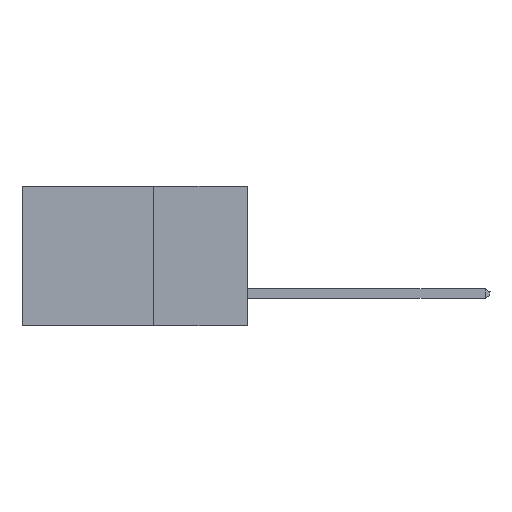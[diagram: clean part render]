
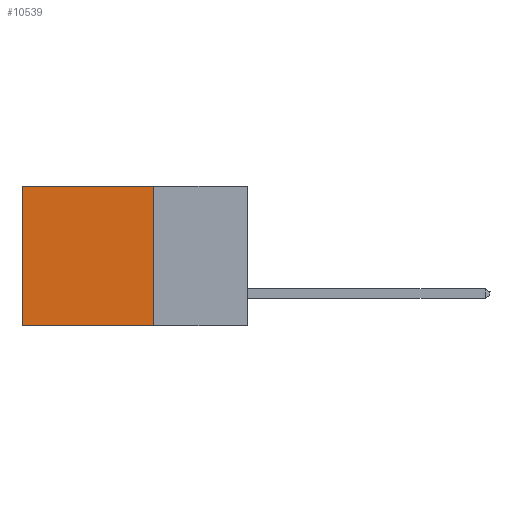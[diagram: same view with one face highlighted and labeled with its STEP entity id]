
A CAD part, left-side view. The second image highlights one B-rep face of the part: STEP entity #10539.
In plain terms, the highlighted planar face has unit normal (-1, 0, 0).
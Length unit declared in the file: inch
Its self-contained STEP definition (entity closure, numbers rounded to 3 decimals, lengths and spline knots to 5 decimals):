
#1441 = CARTESIAN_POINT ( 'NONE',  ( 0.2615, 0.25, -0.37 ) ) ;
#1574 = EDGE_CURVE ( 'NONE', #5538, #5189, #11603, .T. ) ;
#1950 = EDGE_CURVE ( 'NONE', #5538, #12675, #4213, .T. ) ;
#2228 = EDGE_LOOP ( 'NONE', ( #14907, #11228, #4739, #11250 ) ) ;
#2386 = FACE_OUTER_BOUND ( 'NONE', #2228, .T. ) ;
#3394 = CARTESIAN_POINT ( 'NONE',  ( 0.2615, 0.25, 0. ) ) ;
#4213 = LINE ( 'NONE', #5120, #4455 ) ;
#4455 = VECTOR ( 'NONE', #9991, 39.37008 ) ;
#4698 = DIRECTION ( 'NONE',  ( 0., 0., -1. ) ) ;
#4739 = ORIENTED_EDGE ( 'NONE', *, *, #1574, .F. ) ;
#5120 = CARTESIAN_POINT ( 'NONE',  ( 0.2615, 0.25, 0. ) ) ;
#5189 = VERTEX_POINT ( 'NONE', #6951 ) ;
#5538 = VERTEX_POINT ( 'NONE', #3394 ) ;
#6951 = CARTESIAN_POINT ( 'NONE',  ( 0.2615, 0.25, -0.37 ) ) ;
#7607 = DIRECTION ( 'NONE',  ( 0., 1., 0. ) ) ;
#7845 = VERTEX_POINT ( 'NONE', #7915 ) ;
#7915 = CARTESIAN_POINT ( 'NONE',  ( 0.2615, 0.6, -0.37 ) ) ;
#8578 = LINE ( 'NONE', #14483, #9137 ) ;
#9137 = VECTOR ( 'NONE', #10719, 39.37008 ) ;
#9604 = AXIS2_PLACEMENT_3D ( 'NONE', #10703, #13439, #4698 ) ;
#9991 = DIRECTION ( 'NONE',  ( 0., 1., 0. ) ) ;
#10288 = CARTESIAN_POINT ( 'NONE',  ( 0.2615, 0.6, 0. ) ) ;
#10539 = ADVANCED_FACE ( 'NONE', ( #2386 ), #12077, .F. ) ;
#10703 = CARTESIAN_POINT ( 'NONE',  ( 0.2615, 0.25, -0.37 ) ) ;
#10719 = DIRECTION ( 'NONE',  ( 0., 0., -1. ) ) ;
#11228 = ORIENTED_EDGE ( 'NONE', *, *, #13403, .F. ) ;
#11250 = ORIENTED_EDGE ( 'NONE', *, *, #1950, .T. ) ;
#11603 = LINE ( 'NONE', #14154, #12344 ) ;
#11924 = EDGE_CURVE ( 'NONE', #12675, #7845, #8578, .T. ) ;
#12077 = PLANE ( 'NONE',  #9604 ) ;
#12344 = VECTOR ( 'NONE', #15291, 39.37008 ) ;
#12675 = VERTEX_POINT ( 'NONE', #10288 ) ;
#13403 = EDGE_CURVE ( 'NONE', #5189, #7845, #13923, .T. ) ;
#13439 = DIRECTION ( 'NONE',  ( 1., 0., 0. ) ) ;
#13476 = VECTOR ( 'NONE', #7607, 39.37008 ) ;
#13923 = LINE ( 'NONE', #1441, #13476 ) ;
#14154 = CARTESIAN_POINT ( 'NONE',  ( 0.2615, 0.25, -0.37 ) ) ;
#14483 = CARTESIAN_POINT ( 'NONE',  ( 0.2615, 0.6, -0.37 ) ) ;
#14907 = ORIENTED_EDGE ( 'NONE', *, *, #11924, .T. ) ;
#15291 = DIRECTION ( 'NONE',  ( 0., 0., -1. ) ) ;
